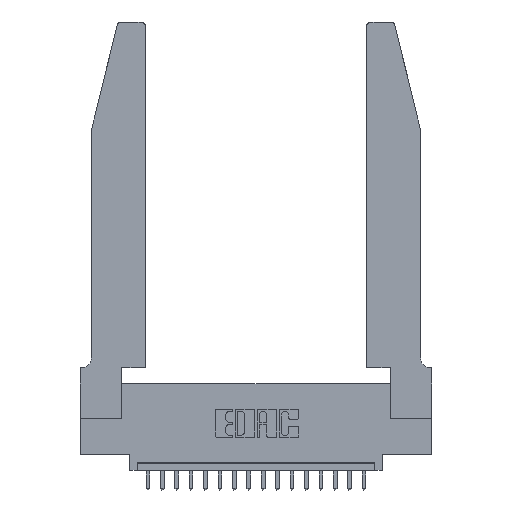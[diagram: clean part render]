
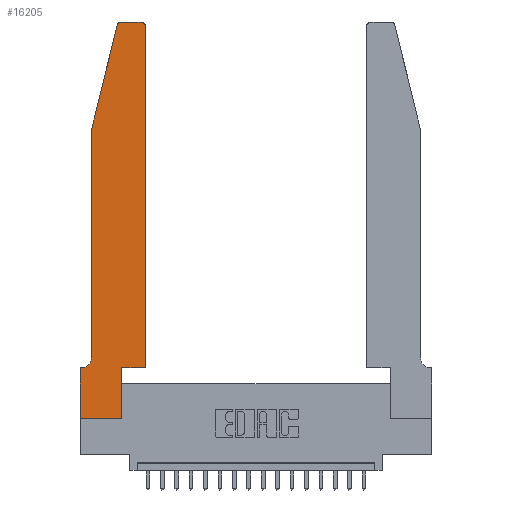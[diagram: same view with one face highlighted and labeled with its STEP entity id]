
A CAD part, top view. The second image highlights one B-rep face of the part: STEP entity #16205.
In plain terms, the highlighted planar face has unit normal (0, 0, 1).
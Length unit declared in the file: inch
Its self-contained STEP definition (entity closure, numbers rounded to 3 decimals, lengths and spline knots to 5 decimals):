
#114 = DIRECTION ( 'NONE',  ( -1., 0., 0. ) ) ;
#161 = EDGE_CURVE ( 'NONE', #15049, #10058, #2821, .T. ) ;
#461 = DIRECTION ( 'NONE',  ( -0.239, -0.971, 0. ) ) ;
#593 = LINE ( 'NONE', #6595, #17829 ) ;
#960 = EDGE_CURVE ( 'NONE', #14658, #8248, #9283, .T. ) ;
#1004 = DIRECTION ( 'NONE',  ( 0., 0., 1. ) ) ;
#1289 = ORIENTED_EDGE ( 'NONE', *, *, #15498, .T. ) ;
#1709 = AXIS2_PLACEMENT_3D ( 'NONE', #13691, #1004, #7242 ) ;
#1840 = DIRECTION ( 'NONE',  ( 0., -1., 0. ) ) ;
#1994 = EDGE_CURVE ( 'NONE', #2153, #15798, #17166, .T. ) ;
#2153 = VERTEX_POINT ( 'NONE', #18995 ) ;
#2247 = CARTESIAN_POINT ( 'NONE',  ( 0.25487, 2.72718, 0.37 ) ) ;
#2306 = DIRECTION ( 'NONE',  ( 0., 0., 1. ) ) ;
#2821 = CIRCLE ( 'NONE', #1709, 0.03 ) ;
#2888 = VECTOR ( 'NONE', #19278, 39.37008 ) ;
#3363 = DIRECTION ( 'NONE',  ( 1., 0., 0. ) ) ;
#4162 = CIRCLE ( 'NONE', #9676, 0.07 ) ;
#4287 = LINE ( 'NONE', #15724, #12164 ) ;
#4353 = CARTESIAN_POINT ( 'NONE',  ( 0.284, 2.75, 0.37 ) ) ;
#4526 = VERTEX_POINT ( 'NONE', #19639 ) ;
#4567 = ORIENTED_EDGE ( 'NONE', *, *, #17678, .T. ) ;
#5309 = AXIS2_PLACEMENT_3D ( 'NONE', #12159, #12199, #18456 ) ;
#5417 = CARTESIAN_POINT ( 'NONE',  ( 0.4205, 2.72, 0.37 ) ) ;
#5426 = LINE ( 'NONE', #8732, #8614 ) ;
#6201 = EDGE_CURVE ( 'NONE', #17417, #14658, #19178, .T. ) ;
#6584 = LINE ( 'NONE', #8446, #2888 ) ;
#6595 = CARTESIAN_POINT ( 'NONE',  ( 0.0755, 2., 0.37 ) ) ;
#6704 = EDGE_CURVE ( 'NONE', #4526, #2153, #4162, .T. ) ;
#6759 = ORIENTED_EDGE ( 'NONE', *, *, #14351, .T. ) ;
#6890 = VECTOR ( 'NONE', #1840, 39.37008 ) ;
#7242 = DIRECTION ( 'NONE',  ( 1., 0., 0. ) ) ;
#7309 = PLANE ( 'NONE',  #5309 ) ;
#7685 = DIRECTION ( 'NONE',  ( -1., 0., 0. ) ) ;
#7813 = CARTESIAN_POINT ( 'NONE',  ( 0., 0.35, 0.37 ) ) ;
#8056 = VERTEX_POINT ( 'NONE', #16925 ) ;
#8248 = VERTEX_POINT ( 'NONE', #17783 ) ;
#8446 = CARTESIAN_POINT ( 'NONE',  ( 0.4505, 0.35, 0.37 ) ) ;
#8614 = VECTOR ( 'NONE', #10395, 39.37008 ) ;
#8732 = CARTESIAN_POINT ( 'NONE',  ( 0.2865, 0.35, 0.37 ) ) ;
#9126 = LINE ( 'NONE', #15165, #10888 ) ;
#9283 = CIRCLE ( 'NONE', #18473, 0.03 ) ;
#9571 = CARTESIAN_POINT ( 'NONE',  ( 0.0755, 0.35, 0.37 ) ) ;
#9676 = AXIS2_PLACEMENT_3D ( 'NONE', #16338, #13142, #19441 ) ;
#9696 = CARTESIAN_POINT ( 'NONE',  ( 0.0755, 2., 0.37 ) ) ;
#9962 = CARTESIAN_POINT ( 'NONE',  ( 0.4505, 0.35, 0.37 ) ) ;
#10058 = VERTEX_POINT ( 'NONE', #2247 ) ;
#10256 = VECTOR ( 'NONE', #7685, 39.37008 ) ;
#10395 = DIRECTION ( 'NONE',  ( 0., 1., 0. ) ) ;
#10408 = CARTESIAN_POINT ( 'NONE',  ( 0., 0., 0.37 ) ) ;
#10748 = LINE ( 'NONE', #18972, #10256 ) ;
#10780 = DIRECTION ( 'NONE',  ( 0., -1., 0. ) ) ;
#10888 = VECTOR ( 'NONE', #10780, 39.37008 ) ;
#11093 = DIRECTION ( 'NONE',  ( 0., 1., 0. ) ) ;
#11497 = VECTOR ( 'NONE', #114, 39.37008 ) ;
#11716 = EDGE_CURVE ( 'NONE', #15798, #18881, #9126, .T. ) ;
#11838 = EDGE_CURVE ( 'NONE', #12488, #4526, #11862, .T. ) ;
#11862 = LINE ( 'NONE', #15814, #6890 ) ;
#12149 = EDGE_LOOP ( 'NONE', ( #17906, #19308, #16693, #18399, #16174, #12297, #19859, #4567, #6759, #1289, #12217, #15908 ) ) ;
#12159 = CARTESIAN_POINT ( 'NONE',  ( 0., 0.35, 0.37 ) ) ;
#12164 = VECTOR ( 'NONE', #3363, 39.37008 ) ;
#12199 = DIRECTION ( 'NONE',  ( 0., 0., 1. ) ) ;
#12217 = ORIENTED_EDGE ( 'NONE', *, *, #6201, .T. ) ;
#12297 = ORIENTED_EDGE ( 'NONE', *, *, #1994, .T. ) ;
#12488 = VERTEX_POINT ( 'NONE', #9696 ) ;
#12991 = FACE_OUTER_BOUND ( 'NONE', #12149, .T. ) ;
#13142 = DIRECTION ( 'NONE',  ( 0., 0., -1. ) ) ;
#13345 = DIRECTION ( 'NONE',  ( 1., 0., 0. ) ) ;
#13381 = CARTESIAN_POINT ( 'NONE',  ( 0.2865, 0., 0.37 ) ) ;
#13691 = CARTESIAN_POINT ( 'NONE',  ( 0.284, 2.72, 0.37 ) ) ;
#14351 = EDGE_CURVE ( 'NONE', #18402, #8056, #5426, .T. ) ;
#14658 = VERTEX_POINT ( 'NONE', #19968 ) ;
#14991 = VECTOR ( 'NONE', #11093, 39.37008 ) ;
#15049 = VERTEX_POINT ( 'NONE', #4353 ) ;
#15165 = CARTESIAN_POINT ( 'NONE',  ( 0., 0., 0.37 ) ) ;
#15498 = EDGE_CURVE ( 'NONE', #8056, #17417, #6584, .T. ) ;
#15724 = CARTESIAN_POINT ( 'NONE',  ( 0., 0., 0.37 ) ) ;
#15798 = VERTEX_POINT ( 'NONE', #7813 ) ;
#15814 = CARTESIAN_POINT ( 'NONE',  ( 0.0755, 2., 0.37 ) ) ;
#15867 = EDGE_CURVE ( 'NONE', #8248, #15049, #10748, .T. ) ;
#15908 = ORIENTED_EDGE ( 'NONE', *, *, #960, .T. ) ;
#16174 = ORIENTED_EDGE ( 'NONE', *, *, #6704, .T. ) ;
#16205 = ADVANCED_FACE ( 'NONE', ( #12991 ), #7309, .T. ) ;
#16338 = CARTESIAN_POINT ( 'NONE',  ( 0.0055, 0.42, 0.37 ) ) ;
#16693 = ORIENTED_EDGE ( 'NONE', *, *, #17243, .T. ) ;
#16925 = CARTESIAN_POINT ( 'NONE',  ( 0.2865, 0.35, 0.37 ) ) ;
#17166 = LINE ( 'NONE', #9571, #11497 ) ;
#17243 = EDGE_CURVE ( 'NONE', #10058, #12488, #593, .T. ) ;
#17417 = VERTEX_POINT ( 'NONE', #9962 ) ;
#17678 = EDGE_CURVE ( 'NONE', #18881, #18402, #4287, .T. ) ;
#17783 = CARTESIAN_POINT ( 'NONE',  ( 0.4205, 2.75, 0.37 ) ) ;
#17829 = VECTOR ( 'NONE', #461, 39.37008 ) ;
#17906 = ORIENTED_EDGE ( 'NONE', *, *, #15867, .T. ) ;
#18399 = ORIENTED_EDGE ( 'NONE', *, *, #11838, .T. ) ;
#18402 = VERTEX_POINT ( 'NONE', #13381 ) ;
#18456 = DIRECTION ( 'NONE',  ( 1., 0., 0. ) ) ;
#18473 = AXIS2_PLACEMENT_3D ( 'NONE', #5417, #2306, #13345 ) ;
#18810 = CARTESIAN_POINT ( 'NONE',  ( 0.4505, 0.35, 0.37 ) ) ;
#18881 = VERTEX_POINT ( 'NONE', #10408 ) ;
#18972 = CARTESIAN_POINT ( 'NONE',  ( 0.2605, 2.75, 0.37 ) ) ;
#18995 = CARTESIAN_POINT ( 'NONE',  ( 0.0055, 0.35, 0.37 ) ) ;
#19178 = LINE ( 'NONE', #18810, #14991 ) ;
#19278 = DIRECTION ( 'NONE',  ( 1., 0., 0. ) ) ;
#19308 = ORIENTED_EDGE ( 'NONE', *, *, #161, .T. ) ;
#19441 = DIRECTION ( 'NONE',  ( -1., 0., 0. ) ) ;
#19639 = CARTESIAN_POINT ( 'NONE',  ( 0.0755, 0.42, 0.37 ) ) ;
#19859 = ORIENTED_EDGE ( 'NONE', *, *, #11716, .T. ) ;
#19968 = CARTESIAN_POINT ( 'NONE',  ( 0.4505, 2.72, 0.37 ) ) ;
